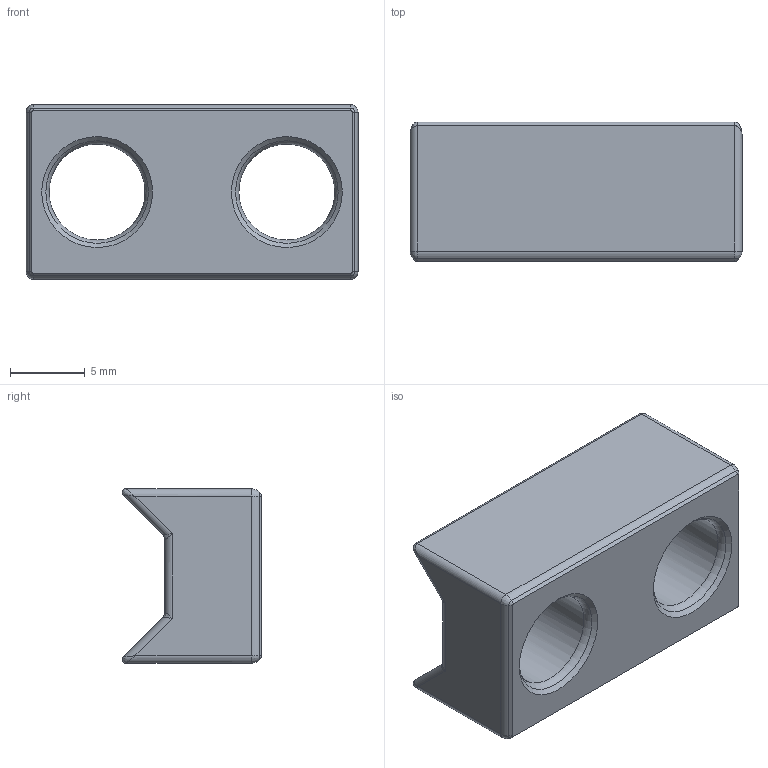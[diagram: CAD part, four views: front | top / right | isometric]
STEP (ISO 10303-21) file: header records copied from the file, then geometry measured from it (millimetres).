
FILE_DESCRIPTION(/* description */ (''),/* implementation_level */ '2;1');
FILE_NAME(/* name */ 'Barrel Retention V Block.step',/* time_stamp */ '2021-10-27T06:44:12-04:00',/* author */ (''),/* organization */ (''),/* preprocessor_version */ 'ST-DEVELOPER v18.1',/* originating_system */ 'Autodesk Translation Framework v10.10.0.1391',/* authorisation */ '');
FILE_SCHEMA (('AUTOMOTIVE_DESIGN { 1 0 10303 214 3 1 1 }'));
Length unit declared in the file: millimetre
Products named in the file (1): Barrel Retention V Block
Bounding box: 22.23 x 9.34 x 11.69 mm (x, y, z)
Volume: 1468.5 mm3; surface area: 1253 mm2
Topology: 1 solids, 1 shells, 107 faces, 246 edges, 136 vertices
Faces by surface type: cylinder 38, bspline 30, plane 19, torus 14, cone 6
Full cylindrical faces by diameter (mm): 3.921 x1, 4.528 x1, 6.426 x2
Entity records: 3518 total; most frequent: CARTESIAN_POINT 1128, DIRECTION 526, ORIENTED_EDGE 476, EDGE_CURVE 238, AXIS2_PLACEMENT_3D 226, VERTEX_POINT 136, CIRCLE 124, EDGE_LOOP 114
